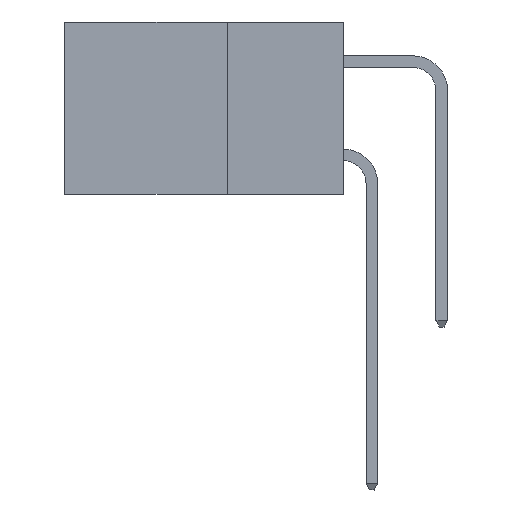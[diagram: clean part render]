
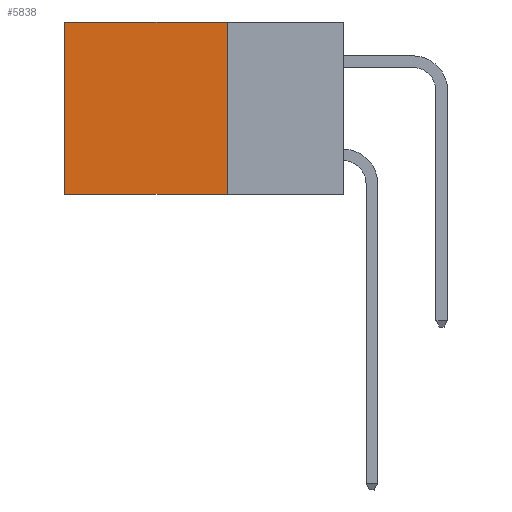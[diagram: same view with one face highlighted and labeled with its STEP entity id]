
A CAD part, left-side view. The second image highlights one B-rep face of the part: STEP entity #5838.
In plain terms, the highlighted planar face has unit normal (-1, 0, 0).
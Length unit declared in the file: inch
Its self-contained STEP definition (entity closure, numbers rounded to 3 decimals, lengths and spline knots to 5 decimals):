
#1516 = VECTOR ( 'NONE', #16520, 39.37008 ) ;
#1563 = CARTESIAN_POINT ( 'NONE',  ( 0.2615, 0.25, -0.37 ) ) ;
#2042 = CARTESIAN_POINT ( 'NONE',  ( 0.2615, 0.6, -0.37 ) ) ;
#2177 = DIRECTION ( 'NONE',  ( 0., 0., -1. ) ) ;
#2383 = CARTESIAN_POINT ( 'NONE',  ( 0.2615, 0.6, -0.37 ) ) ;
#4182 = LINE ( 'NONE', #5993, #21136 ) ;
#4965 = ORIENTED_EDGE ( 'NONE', *, *, #5263, .F. ) ;
#5101 = CARTESIAN_POINT ( 'NONE',  ( 0.2615, 0.25, 0. ) ) ;
#5263 = EDGE_CURVE ( 'NONE', #12572, #20657, #4182, .T. ) ;
#5838 = ADVANCED_FACE ( 'NONE', ( #14816 ), #25589, .F. ) ;
#5993 = CARTESIAN_POINT ( 'NONE',  ( 0.2615, 0.25, -0.37 ) ) ;
#6469 = ORIENTED_EDGE ( 'NONE', *, *, #20236, .T. ) ;
#8483 = EDGE_CURVE ( 'NONE', #22689, #24055, #23621, .T. ) ;
#9349 = ORIENTED_EDGE ( 'NONE', *, *, #8483, .T. ) ;
#9802 = CARTESIAN_POINT ( 'NONE',  ( 0.2615, 0.25, -0.37 ) ) ;
#12300 = CARTESIAN_POINT ( 'NONE',  ( 0.2615, 0.6, 0. ) ) ;
#12572 = VERTEX_POINT ( 'NONE', #9802 ) ;
#14816 = FACE_OUTER_BOUND ( 'NONE', #17255, .T. ) ;
#14829 = DIRECTION ( 'NONE',  ( 0., 1., 0. ) ) ;
#15614 = DIRECTION ( 'NONE',  ( 0., 1., 0. ) ) ;
#16066 = VECTOR ( 'NONE', #15614, 39.37008 ) ;
#16520 = DIRECTION ( 'NONE',  ( 0., 0., -1. ) ) ;
#17255 = EDGE_LOOP ( 'NONE', ( #6469, #4965, #18562, #9349 ) ) ;
#18562 = ORIENTED_EDGE ( 'NONE', *, *, #24443, .F. ) ;
#19253 = DIRECTION ( 'NONE',  ( 0., 0., -1. ) ) ;
#19826 = AXIS2_PLACEMENT_3D ( 'NONE', #21189, #23246, #19253 ) ;
#19986 = VECTOR ( 'NONE', #2177, 39.37008 ) ;
#20236 = EDGE_CURVE ( 'NONE', #24055, #20657, #20998, .T. ) ;
#20657 = VERTEX_POINT ( 'NONE', #2383 ) ;
#20998 = LINE ( 'NONE', #2042, #19986 ) ;
#21136 = VECTOR ( 'NONE', #14829, 39.37008 ) ;
#21189 = CARTESIAN_POINT ( 'NONE',  ( 0.2615, 0.25, -0.37 ) ) ;
#22411 = CARTESIAN_POINT ( 'NONE',  ( 0.2615, 0.25, 0. ) ) ;
#22594 = LINE ( 'NONE', #1563, #1516 ) ;
#22689 = VERTEX_POINT ( 'NONE', #22411 ) ;
#23246 = DIRECTION ( 'NONE',  ( 1., 0., 0. ) ) ;
#23621 = LINE ( 'NONE', #5101, #16066 ) ;
#24055 = VERTEX_POINT ( 'NONE', #12300 ) ;
#24443 = EDGE_CURVE ( 'NONE', #22689, #12572, #22594, .T. ) ;
#25589 = PLANE ( 'NONE',  #19826 ) ;
